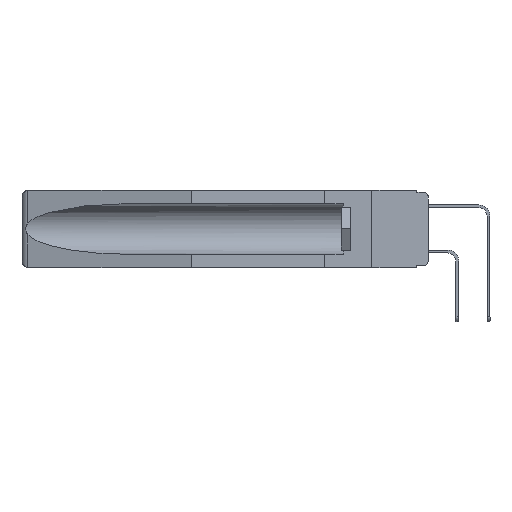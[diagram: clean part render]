
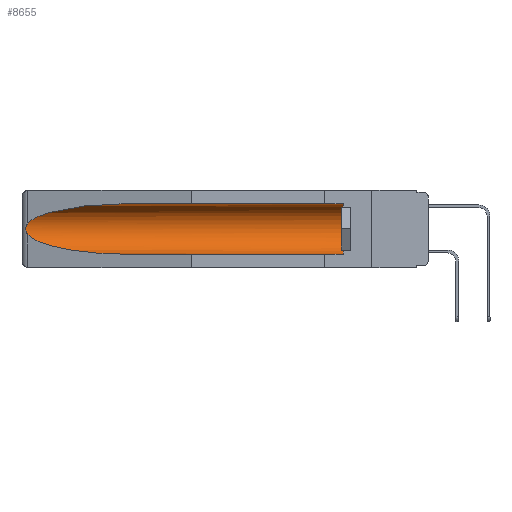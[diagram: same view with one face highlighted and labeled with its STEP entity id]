
A CAD part, left-side view. The second image highlights one B-rep face of the part: STEP entity #8655.
In plain terms, the highlighted cylindrical face has radius 2.857 mm (diameter 5.715 mm), a partial arc.
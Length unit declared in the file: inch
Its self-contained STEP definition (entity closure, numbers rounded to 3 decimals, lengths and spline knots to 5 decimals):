
#160 = DIRECTION ( 'NONE',  ( 0., 0., 1. ) ) ;
#641 =( BOUNDED_CURVE ( )  B_SPLINE_CURVE ( 3, ( #19186, #18927, #19054, #2264 ),
 .UNSPECIFIED., .F., .T. ) 
 B_SPLINE_CURVE_WITH_KNOTS ( ( 4, 4 ),
 ( 4.71239, 6.08839 ),
 .UNSPECIFIED. ) 
 CURVE ( )  GEOMETRIC_REPRESENTATION_ITEM ( )  RATIONAL_B_SPLINE_CURVE ( ( 1., 0.848, 0.848, 1. ) ) 
 REPRESENTATION_ITEM ( '' )  );
#1007 = DIRECTION ( 'NONE',  ( 0., 1., 0. ) ) ;
#1317 = LINE ( 'NONE', #17996, #16197 ) ;
#2264 = CARTESIAN_POINT ( 'NONE',  ( 0.26537, 1.52718, -0.14972 ) ) ;
#2447 = EDGE_CURVE ( 'NONE', #14425, #13777, #6642, .T. ) ;
#2526 = B_SPLINE_CURVE_WITH_KNOTS ( 'NONE', 3,
 ( #10345, #8726, #23816, #16391, #3780, #8974, #18362, #7475, #5262, #15008 ),
 .UNSPECIFIED., .F., .F.,
 ( 4, 2, 2, 2, 4 ),
 ( 0., 0.00029, 0.00058, 0.00087, 0.00117 ),
 .UNSPECIFIED. ) ;
#2970 = AXIS2_PLACEMENT_3D ( 'NONE', #6193, #1007, #11869 ) ;
#3230 = ORIENTED_EDGE ( 'NONE', *, *, #2447, .T. ) ;
#3780 = CARTESIAN_POINT ( 'NONE',  ( 0.2675, 1.53308, -0.16763 ) ) ;
#4780 = ORIENTED_EDGE ( 'NONE', *, *, #21452, .T. ) ;
#5262 = CARTESIAN_POINT ( 'NONE',  ( 0.26597, 1.5296, -0.19026 ) ) ;
#6193 = CARTESIAN_POINT ( 'NONE',  ( 0.155, -0.30754, -0.1715 ) ) ;
#6642 = LINE ( 'NONE', #23822, #10205 ) ;
#6835 = AXIS2_PLACEMENT_3D ( 'NONE', #9535, #17077, #160 ) ;
#6890 = DIRECTION ( 'NONE',  ( 0., 1., 0. ) ) ;
#7475 = CARTESIAN_POINT ( 'NONE',  ( 0.26655, 1.53094, -0.18657 ) ) ;
#8655 = ADVANCED_FACE ( 'NONE', ( #12126 ), #19659, .F. ) ;
#8726 = CARTESIAN_POINT ( 'NONE',  ( 0.26597, 1.52961, -0.15275 ) ) ;
#8974 = CARTESIAN_POINT ( 'NONE',  ( 0.2675, 1.53308, -0.17534 ) ) ;
#9535 = CARTESIAN_POINT ( 'NONE',  ( 0.155, 0.126, -0.1715 ) ) ;
#10205 = VECTOR ( 'NONE', #6890, 39.37008 ) ;
#10345 = CARTESIAN_POINT ( 'NONE',  ( 0.26537, 1.52718, -0.14972 ) ) ;
#11520 = CARTESIAN_POINT ( 'NONE',  ( 0.26537, 1.52718, -0.19328 ) ) ;
#11718 = VERTEX_POINT ( 'NONE', #17431 ) ;
#11798 = ORIENTED_EDGE ( 'NONE', *, *, #22614, .T. ) ;
#11869 = DIRECTION ( 'NONE',  ( 0., 0., 1. ) ) ;
#12126 = FACE_OUTER_BOUND ( 'NONE', #15305, .T. ) ;
#12347 = EDGE_CURVE ( 'NONE', #21993, #17623, #1317, .T. ) ;
#13720 = ORIENTED_EDGE ( 'NONE', *, *, #12347, .F. ) ;
#13746 = CARTESIAN_POINT ( 'NONE',  ( 0.25451, 1.48313, -0.24835 ) ) ;
#13753 = VERTEX_POINT ( 'NONE', #16533 ) ;
#13777 = VERTEX_POINT ( 'NONE', #22238 ) ;
#13942 = CIRCLE ( 'NONE', #6835, 0.1125 ) ;
#14425 = VERTEX_POINT ( 'NONE', #21776 ) ;
#15008 = CARTESIAN_POINT ( 'NONE',  ( 0.26537, 1.52718, -0.19328 ) ) ;
#15107 = CARTESIAN_POINT ( 'NONE',  ( 0.21114, 1.30732, -0.284 ) ) ;
#15305 = EDGE_LOOP ( 'NONE', ( #23954, #24311, #11798, #13720, #4780, #3230 ) ) ;
#16197 = VECTOR ( 'NONE', #16385, 39.37008 ) ;
#16385 = DIRECTION ( 'NONE',  ( 0., 1., 0. ) ) ;
#16391 = CARTESIAN_POINT ( 'NONE',  ( 0.2673, 1.5327, -0.16383 ) ) ;
#16533 = CARTESIAN_POINT ( 'NONE',  ( 0.26537, 1.52718, -0.19328 ) ) ;
#16654 = CARTESIAN_POINT ( 'NONE',  ( 0.155, 0.126, -0.284 ) ) ;
#17077 = DIRECTION ( 'NONE',  ( 0., -1., 0. ) ) ;
#17431 = CARTESIAN_POINT ( 'NONE',  ( 0.26537, 1.52718, -0.14972 ) ) ;
#17623 = VERTEX_POINT ( 'NONE', #18498 ) ;
#17996 = CARTESIAN_POINT ( 'NONE',  ( 0.155, -0.30754, -0.284 ) ) ;
#18362 = CARTESIAN_POINT ( 'NONE',  ( 0.2673, 1.53269, -0.17917 ) ) ;
#18498 = CARTESIAN_POINT ( 'NONE',  ( 0.155, 1.07973, -0.284 ) ) ;
#18927 = CARTESIAN_POINT ( 'NONE',  ( 0.21114, 1.30732, -0.059 ) ) ;
#19054 = CARTESIAN_POINT ( 'NONE',  ( 0.25451, 1.48313, -0.09465 ) ) ;
#19186 = CARTESIAN_POINT ( 'NONE',  ( 0.155, 1.07973, -0.059 ) ) ;
#19432 = CARTESIAN_POINT ( 'NONE',  ( 0.155, 1.07973, -0.284 ) ) ;
#19659 = CYLINDRICAL_SURFACE ( 'NONE', #2970, 0.1125 ) ;
#20099 = EDGE_CURVE ( 'NONE', #13777, #11718, #641, .T. ) ;
#20724 = EDGE_CURVE ( 'NONE', #11718, #13753, #2526, .T. ) ;
#20837 =( BOUNDED_CURVE ( )  B_SPLINE_CURVE ( 3, ( #11520, #13746, #15107, #19432 ),
 .UNSPECIFIED., .F., .T. ) 
 B_SPLINE_CURVE_WITH_KNOTS ( ( 4, 4 ),
 ( 0.1948, 1.5708 ),
 .UNSPECIFIED. ) 
 CURVE ( )  GEOMETRIC_REPRESENTATION_ITEM ( )  RATIONAL_B_SPLINE_CURVE ( ( 1., 0.848, 0.848, 1. ) ) 
 REPRESENTATION_ITEM ( '' )  );
#21452 = EDGE_CURVE ( 'NONE', #21993, #14425, #13942, .T. ) ;
#21776 = CARTESIAN_POINT ( 'NONE',  ( 0.155, 0.126, -0.059 ) ) ;
#21993 = VERTEX_POINT ( 'NONE', #16654 ) ;
#22238 = CARTESIAN_POINT ( 'NONE',  ( 0.155, 1.07973, -0.059 ) ) ;
#22614 = EDGE_CURVE ( 'NONE', #13753, #17623, #20837, .T. ) ;
#23816 = CARTESIAN_POINT ( 'NONE',  ( 0.26654, 1.53092, -0.15636 ) ) ;
#23822 = CARTESIAN_POINT ( 'NONE',  ( 0.155, -0.30754, -0.059 ) ) ;
#23954 = ORIENTED_EDGE ( 'NONE', *, *, #20099, .T. ) ;
#24311 = ORIENTED_EDGE ( 'NONE', *, *, #20724, .T. ) ;
